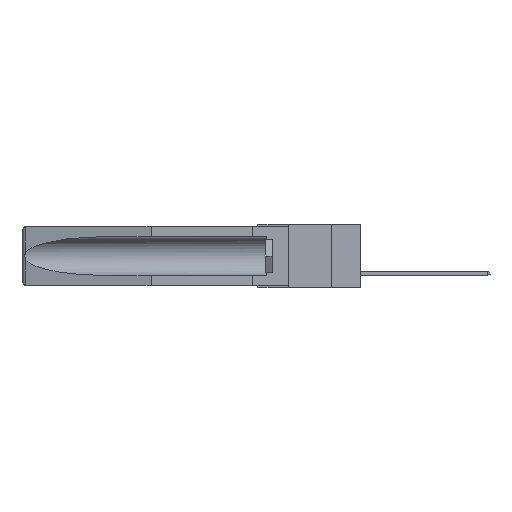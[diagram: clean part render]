
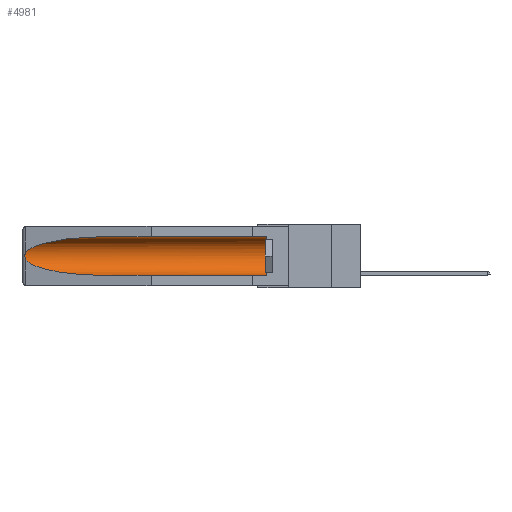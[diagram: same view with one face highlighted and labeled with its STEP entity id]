
A CAD part, left-side view. The second image highlights one B-rep face of the part: STEP entity #4981.
In plain terms, the highlighted cylindrical face has radius 2.857 mm (diameter 5.715 mm), a partial arc.
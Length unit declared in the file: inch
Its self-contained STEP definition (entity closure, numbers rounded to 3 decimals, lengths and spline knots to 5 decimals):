
#258 = ORIENTED_EDGE ( 'NONE', *, *, #2671, .T. ) ;
#621 = DIRECTION ( 'NONE',  ( 0., 0., 1. ) ) ;
#857 = CARTESIAN_POINT ( 'NONE',  ( 0.155, -0.30754, -0.1715 ) ) ;
#875 = CARTESIAN_POINT ( 'NONE',  ( 0.26654, 1.53092, -0.15636 ) ) ;
#879 = CARTESIAN_POINT ( 'NONE',  ( 0.26537, 1.52718, -0.19328 ) ) ;
#987 = CARTESIAN_POINT ( 'NONE',  ( 0.26655, 1.53094, -0.18657 ) ) ;
#1115 = CARTESIAN_POINT ( 'NONE',  ( 0.26537, 1.52718, -0.19328 ) ) ;
#1328 = CARTESIAN_POINT ( 'NONE',  ( 0.26537, 1.52718, -0.14972 ) ) ;
#1333 = CYLINDRICAL_SURFACE ( 'NONE', #2375, 0.1125 ) ;
#1510 = VERTEX_POINT ( 'NONE', #17996 ) ;
#1525 = CARTESIAN_POINT ( 'NONE',  ( 0.26537, 1.52718, -0.14972 ) ) ;
#1641 = EDGE_CURVE ( 'NONE', #9477, #8860, #13906, .T. ) ;
#1767 = EDGE_CURVE ( 'NONE', #8860, #14875, #11946, .T. ) ;
#1801 = CARTESIAN_POINT ( 'NONE',  ( 0.155, -0.30754, -0.284 ) ) ;
#1844 = VECTOR ( 'NONE', #3138, 39.37008 ) ;
#2002 = CIRCLE ( 'NONE', #14807, 0.1125 ) ;
#2156 = ORIENTED_EDGE ( 'NONE', *, *, #1767, .T. ) ;
#2348 = CARTESIAN_POINT ( 'NONE',  ( 0.25451, 1.48313, -0.24835 ) ) ;
#2375 = AXIS2_PLACEMENT_3D ( 'NONE', #857, #9623, #18138 ) ;
#2671 = EDGE_CURVE ( 'NONE', #1510, #9477, #13344, .T. ) ;
#2712 = LINE ( 'NONE', #1801, #1844 ) ;
#3138 = DIRECTION ( 'NONE',  ( 0., 1., 0. ) ) ;
#3440 = CARTESIAN_POINT ( 'NONE',  ( 0.26597, 1.52961, -0.15275 ) ) ;
#3801 = CARTESIAN_POINT ( 'NONE',  ( 0.2675, 1.53308, -0.16763 ) ) ;
#4044 = CARTESIAN_POINT ( 'NONE',  ( 0.155, 1.07973, -0.059 ) ) ;
#4761 = CARTESIAN_POINT ( 'NONE',  ( 0.26537, 1.52718, -0.14972 ) ) ;
#4834 = EDGE_CURVE ( 'NONE', #17926, #1510, #2002, .T. ) ;
#4930 = CARTESIAN_POINT ( 'NONE',  ( 0.155, -0.30754, -0.059 ) ) ;
#4981 = ADVANCED_FACE ( 'NONE', ( #16520 ), #1333, .F. ) ;
#4987 = DIRECTION ( 'NONE',  ( 0., -1., 0. ) ) ;
#5002 = CARTESIAN_POINT ( 'NONE',  ( 0.2673, 1.5327, -0.16383 ) ) ;
#5319 = VECTOR ( 'NONE', #17775, 39.37008 ) ;
#5350 = CARTESIAN_POINT ( 'NONE',  ( 0.21114, 1.30732, -0.284 ) ) ;
#5472 = VERTEX_POINT ( 'NONE', #6068 ) ;
#5888 = CARTESIAN_POINT ( 'NONE',  ( 0.21114, 1.30732, -0.059 ) ) ;
#6068 = CARTESIAN_POINT ( 'NONE',  ( 0.155, 1.07973, -0.284 ) ) ;
#6295 = CARTESIAN_POINT ( 'NONE',  ( 0.155, 0.126, -0.1715 ) ) ;
#7335 = ORIENTED_EDGE ( 'NONE', *, *, #10616, .T. ) ;
#7437 = CARTESIAN_POINT ( 'NONE',  ( 0.155, 0.126, -0.284 ) ) ;
#8153 = CARTESIAN_POINT ( 'NONE',  ( 0.26597, 1.5296, -0.19026 ) ) ;
#8799 = CARTESIAN_POINT ( 'NONE',  ( 0.155, 1.07973, -0.059 ) ) ;
#8860 = VERTEX_POINT ( 'NONE', #1328 ) ;
#9477 = VERTEX_POINT ( 'NONE', #4044 ) ;
#9520 = CARTESIAN_POINT ( 'NONE',  ( 0.2673, 1.53269, -0.17917 ) ) ;
#9623 = DIRECTION ( 'NONE',  ( 0., 1., 0. ) ) ;
#10613 = ORIENTED_EDGE ( 'NONE', *, *, #4834, .T. ) ;
#10616 = EDGE_CURVE ( 'NONE', #14875, #5472, #13582, .T. ) ;
#11209 = CARTESIAN_POINT ( 'NONE',  ( 0.2675, 1.53308, -0.17534 ) ) ;
#11315 = EDGE_CURVE ( 'NONE', #17926, #5472, #2712, .T. ) ;
#11946 = B_SPLINE_CURVE_WITH_KNOTS ( 'NONE', 3,
 ( #4761, #3440, #875, #5002, #3801, #11209, #9520, #987, #8153, #1115 ),
 .UNSPECIFIED., .F., .F.,
 ( 4, 2, 2, 2, 4 ),
 ( 0., 0.00029, 0.00058, 0.00087, 0.00117 ),
 .UNSPECIFIED. ) ;
#12396 = ORIENTED_EDGE ( 'NONE', *, *, #11315, .F. ) ;
#13038 = CARTESIAN_POINT ( 'NONE',  ( 0.25451, 1.48313, -0.09465 ) ) ;
#13274 = EDGE_LOOP ( 'NONE', ( #15478, #2156, #7335, #12396, #10613, #258 ) ) ;
#13344 = LINE ( 'NONE', #4930, #5319 ) ;
#13582 =( BOUNDED_CURVE ( )  B_SPLINE_CURVE ( 3, ( #16522, #2348, #5350, #13872 ),
 .UNSPECIFIED., .F., .F. ) 
 B_SPLINE_CURVE_WITH_KNOTS ( ( 4, 4 ),
 ( 0.1948, 1.5708 ),
 .UNSPECIFIED. ) 
 CURVE ( )  GEOMETRIC_REPRESENTATION_ITEM ( )  RATIONAL_B_SPLINE_CURVE ( ( 1., 0.848, 0.848, 1. ) ) 
 REPRESENTATION_ITEM ( '' )  );
#13872 = CARTESIAN_POINT ( 'NONE',  ( 0.155, 1.07973, -0.284 ) ) ;
#13906 =( BOUNDED_CURVE ( )  B_SPLINE_CURVE ( 3, ( #8799, #5888, #13038, #1525 ),
 .UNSPECIFIED., .F., .F. ) 
 B_SPLINE_CURVE_WITH_KNOTS ( ( 4, 4 ),
 ( 4.71239, 6.08839 ),
 .UNSPECIFIED. ) 
 CURVE ( )  GEOMETRIC_REPRESENTATION_ITEM ( )  RATIONAL_B_SPLINE_CURVE ( ( 1., 0.848, 0.848, 1. ) ) 
 REPRESENTATION_ITEM ( '' )  );
#14807 = AXIS2_PLACEMENT_3D ( 'NONE', #6295, #4987, #621 ) ;
#14875 = VERTEX_POINT ( 'NONE', #879 ) ;
#15478 = ORIENTED_EDGE ( 'NONE', *, *, #1641, .T. ) ;
#16520 = FACE_OUTER_BOUND ( 'NONE', #13274, .T. ) ;
#16522 = CARTESIAN_POINT ( 'NONE',  ( 0.26537, 1.52718, -0.19328 ) ) ;
#17775 = DIRECTION ( 'NONE',  ( 0., 1., 0. ) ) ;
#17926 = VERTEX_POINT ( 'NONE', #7437 ) ;
#17996 = CARTESIAN_POINT ( 'NONE',  ( 0.155, 0.126, -0.059 ) ) ;
#18138 = DIRECTION ( 'NONE',  ( 0., 0., 1. ) ) ;
